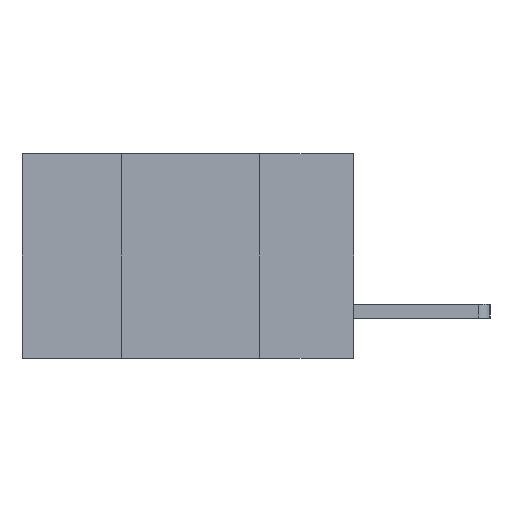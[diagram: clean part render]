
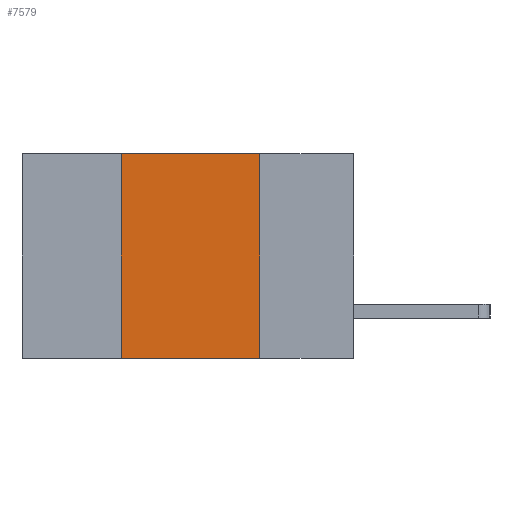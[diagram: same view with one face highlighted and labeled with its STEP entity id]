
A CAD part, left-side view. The second image highlights one B-rep face of the part: STEP entity #7579.
In plain terms, the highlighted planar face has unit normal (-1, 0, 0).
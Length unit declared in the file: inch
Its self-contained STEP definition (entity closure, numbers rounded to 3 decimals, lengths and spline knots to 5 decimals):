
#200 = CARTESIAN_POINT ( 'NONE',  ( 0., 0.42, 0. ) ) ;
#755 = CARTESIAN_POINT ( 'NONE',  ( 0., 0.17, 0. ) ) ;
#958 = CARTESIAN_POINT ( 'NONE',  ( 0., 0.42, -0.37 ) ) ;
#1025 = AXIS2_PLACEMENT_3D ( 'NONE', #6243, #2967, #4689 ) ;
#1238 = FACE_OUTER_BOUND ( 'NONE', #8453, .T. ) ;
#1741 = LINE ( 'NONE', #755, #3848 ) ;
#2002 = ORIENTED_EDGE ( 'NONE', *, *, #2421, .T. ) ;
#2421 = EDGE_CURVE ( 'NONE', #3842, #6609, #10137, .T. ) ;
#2429 = VERTEX_POINT ( 'NONE', #7682 ) ;
#2967 = DIRECTION ( 'NONE',  ( 1., 0., 0. ) ) ;
#3162 = CARTESIAN_POINT ( 'NONE',  ( 0., 0.6, -0.37 ) ) ;
#3842 = VERTEX_POINT ( 'NONE', #958 ) ;
#3848 = VECTOR ( 'NONE', #11284, 39.37008 ) ;
#4163 = DIRECTION ( 'NONE',  ( 0., -1., 0. ) ) ;
#4282 = LINE ( 'NONE', #7760, #4389 ) ;
#4389 = VECTOR ( 'NONE', #10395, 39.37008 ) ;
#4525 = PLANE ( 'NONE',  #1025 ) ;
#4689 = DIRECTION ( 'NONE',  ( 0., 0., -1. ) ) ;
#4966 = LINE ( 'NONE', #8507, #7393 ) ;
#5253 = EDGE_CURVE ( 'NONE', #3842, #10884, #4282, .T. ) ;
#5595 = EDGE_CURVE ( 'NONE', #2429, #6609, #1741, .T. ) ;
#5797 = VECTOR ( 'NONE', #11212, 39.37008 ) ;
#6112 = ORIENTED_EDGE ( 'NONE', *, *, #5595, .F. ) ;
#6243 = CARTESIAN_POINT ( 'NONE',  ( 0., 0.6, 0. ) ) ;
#6609 = VERTEX_POINT ( 'NONE', #6841 ) ;
#6841 = CARTESIAN_POINT ( 'NONE',  ( 0., 0.17, -0.37 ) ) ;
#7393 = VECTOR ( 'NONE', #4163, 39.37008 ) ;
#7579 = ADVANCED_FACE ( 'NONE', ( #1238 ), #4525, .F. ) ;
#7682 = CARTESIAN_POINT ( 'NONE',  ( 0., 0.17, 0. ) ) ;
#7760 = CARTESIAN_POINT ( 'NONE',  ( 0., 0.42, 0. ) ) ;
#8069 = ORIENTED_EDGE ( 'NONE', *, *, #9368, .F. ) ;
#8453 = EDGE_LOOP ( 'NONE', ( #6112, #8069, #9548, #2002 ) ) ;
#8507 = CARTESIAN_POINT ( 'NONE',  ( 0., 0.6, 0. ) ) ;
#9368 = EDGE_CURVE ( 'NONE', #10884, #2429, #4966, .T. ) ;
#9548 = ORIENTED_EDGE ( 'NONE', *, *, #5253, .F. ) ;
#10137 = LINE ( 'NONE', #3162, #5797 ) ;
#10395 = DIRECTION ( 'NONE',  ( 0., 0., 1. ) ) ;
#10884 = VERTEX_POINT ( 'NONE', #200 ) ;
#11212 = DIRECTION ( 'NONE',  ( 0., -1., 0. ) ) ;
#11284 = DIRECTION ( 'NONE',  ( 0., 0., -1. ) ) ;
